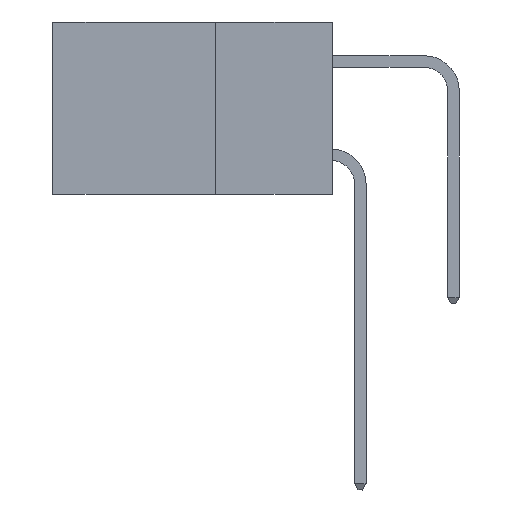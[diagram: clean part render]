
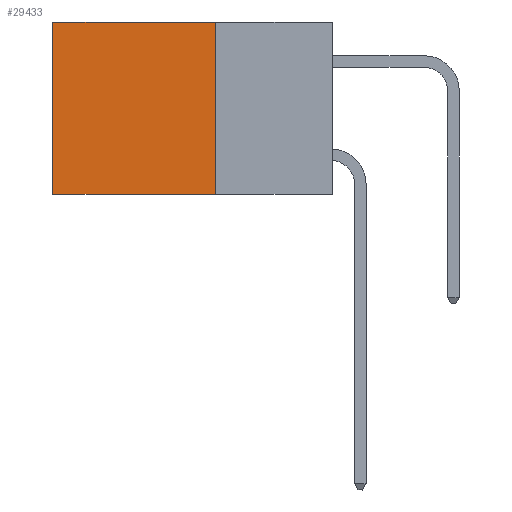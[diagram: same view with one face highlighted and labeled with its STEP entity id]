
A CAD part, left-side view. The second image highlights one B-rep face of the part: STEP entity #29433.
In plain terms, the highlighted planar face has unit normal (-1, 0, 0).
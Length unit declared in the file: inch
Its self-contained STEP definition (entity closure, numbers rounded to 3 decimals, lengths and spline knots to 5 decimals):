
#459 = VECTOR ( 'NONE', #14964, 39.37008 ) ;
#1390 = EDGE_CURVE ( 'NONE', #17226, #5010, #2133, .T. ) ;
#1703 = DIRECTION ( 'NONE',  ( 1., 0., 0. ) ) ;
#1722 = VECTOR ( 'NONE', #20905, 39.37008 ) ;
#2133 = LINE ( 'NONE', #7432, #1722 ) ;
#3823 = DIRECTION ( 'NONE',  ( 0., 1., 0. ) ) ;
#4549 = LINE ( 'NONE', #6400, #16406 ) ;
#4868 = CARTESIAN_POINT ( 'NONE',  ( 0.298, 0.25, 0. ) ) ;
#4965 = CARTESIAN_POINT ( 'NONE',  ( 0.298, 0.6, 0. ) ) ;
#5010 = VERTEX_POINT ( 'NONE', #29529 ) ;
#5573 = CARTESIAN_POINT ( 'NONE',  ( 0.298, 0.6, 0. ) ) ;
#6400 = CARTESIAN_POINT ( 'NONE',  ( 0.298, 0.25, -0.37 ) ) ;
#7432 = CARTESIAN_POINT ( 'NONE',  ( 0.298, 0.25, 0. ) ) ;
#7718 = VECTOR ( 'NONE', #18208, 39.37008 ) ;
#9805 = DIRECTION ( 'NONE',  ( 0., 0., -1. ) ) ;
#10035 = EDGE_CURVE ( 'NONE', #17226, #13928, #26989, .T. ) ;
#13928 = VERTEX_POINT ( 'NONE', #5573 ) ;
#14964 = DIRECTION ( 'NONE',  ( 0., 1., 0. ) ) ;
#15641 = PLANE ( 'NONE',  #29240 ) ;
#16406 = VECTOR ( 'NONE', #3823, 39.37008 ) ;
#17226 = VERTEX_POINT ( 'NONE', #23161 ) ;
#17671 = VERTEX_POINT ( 'NONE', #31211 ) ;
#18208 = DIRECTION ( 'NONE',  ( 0., 0., -1. ) ) ;
#19129 = LINE ( 'NONE', #4965, #7718 ) ;
#20742 = EDGE_LOOP ( 'NONE', ( #27173, #25153, #22426, #24766 ) ) ;
#20905 = DIRECTION ( 'NONE',  ( 0., 0., -1. ) ) ;
#22426 = ORIENTED_EDGE ( 'NONE', *, *, #1390, .F. ) ;
#23161 = CARTESIAN_POINT ( 'NONE',  ( 0.298, 0.25, 0. ) ) ;
#24766 = ORIENTED_EDGE ( 'NONE', *, *, #10035, .T. ) ;
#25102 = EDGE_CURVE ( 'NONE', #13928, #17671, #19129, .T. ) ;
#25153 = ORIENTED_EDGE ( 'NONE', *, *, #28504, .F. ) ;
#26989 = LINE ( 'NONE', #31069, #459 ) ;
#27173 = ORIENTED_EDGE ( 'NONE', *, *, #25102, .T. ) ;
#28504 = EDGE_CURVE ( 'NONE', #5010, #17671, #4549, .T. ) ;
#28930 = FACE_OUTER_BOUND ( 'NONE', #20742, .T. ) ;
#29240 = AXIS2_PLACEMENT_3D ( 'NONE', #4868, #1703, #9805 ) ;
#29433 = ADVANCED_FACE ( 'NONE', ( #28930 ), #15641, .F. ) ;
#29529 = CARTESIAN_POINT ( 'NONE',  ( 0.298, 0.25, -0.37 ) ) ;
#31069 = CARTESIAN_POINT ( 'NONE',  ( 0.298, 0.25, 0. ) ) ;
#31211 = CARTESIAN_POINT ( 'NONE',  ( 0.298, 0.6, -0.37 ) ) ;
